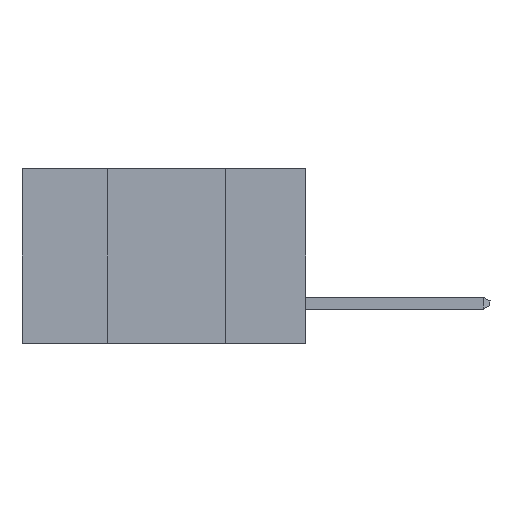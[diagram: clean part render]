
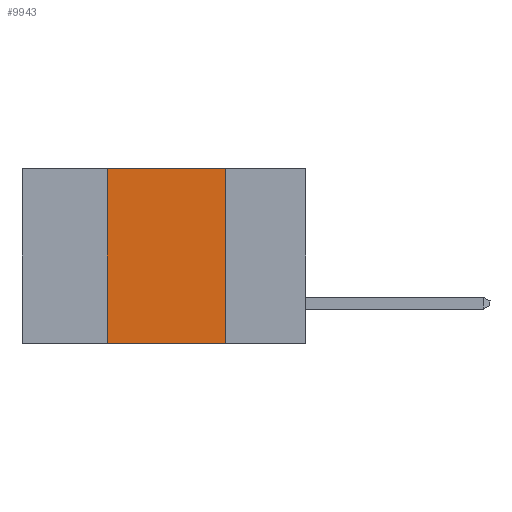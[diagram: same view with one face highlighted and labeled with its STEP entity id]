
A CAD part, left-side view. The second image highlights one B-rep face of the part: STEP entity #9943.
In plain terms, the highlighted planar face has unit normal (-1, 0, 0).
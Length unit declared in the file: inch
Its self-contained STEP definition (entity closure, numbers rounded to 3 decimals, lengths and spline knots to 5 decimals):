
#151 = DIRECTION ( 'NONE',  ( 0., -1., 0. ) ) ;
#464 = EDGE_CURVE ( 'NONE', #7563, #9690, #780, .T. ) ;
#780 = LINE ( 'NONE', #4420, #4636 ) ;
#923 = CARTESIAN_POINT ( 'NONE',  ( 0., 0.17, 0. ) ) ;
#1298 = ORIENTED_EDGE ( 'NONE', *, *, #4960, .F. ) ;
#1433 = EDGE_CURVE ( 'NONE', #7563, #1590, #11849, .T. ) ;
#1549 = CARTESIAN_POINT ( 'NONE',  ( 0., 0.42, -0.37 ) ) ;
#1590 = VERTEX_POINT ( 'NONE', #11187 ) ;
#2091 = AXIS2_PLACEMENT_3D ( 'NONE', #10348, #4934, #11356 ) ;
#2111 = PLANE ( 'NONE',  #2091 ) ;
#2877 = ORIENTED_EDGE ( 'NONE', *, *, #464, .F. ) ;
#3381 = CARTESIAN_POINT ( 'NONE',  ( 0., 0.42, 0. ) ) ;
#3438 = LINE ( 'NONE', #4391, #10645 ) ;
#3635 = VERTEX_POINT ( 'NONE', #923 ) ;
#4286 = VECTOR ( 'NONE', #6633, 39.37008 ) ;
#4391 = CARTESIAN_POINT ( 'NONE',  ( 0., 0.17, -0.37 ) ) ;
#4420 = CARTESIAN_POINT ( 'NONE',  ( 0., 0.42, -0.37 ) ) ;
#4636 = VECTOR ( 'NONE', #9963, 39.37008 ) ;
#4669 = EDGE_CURVE ( 'NONE', #9690, #3635, #11024, .T. ) ;
#4934 = DIRECTION ( 'NONE',  ( 1., 0., 0. ) ) ;
#4960 = EDGE_CURVE ( 'NONE', #3635, #1590, #3438, .T. ) ;
#5655 = ORIENTED_EDGE ( 'NONE', *, *, #1433, .T. ) ;
#6633 = DIRECTION ( 'NONE',  ( 0., -1., 0. ) ) ;
#7159 = DIRECTION ( 'NONE',  ( 0., 0., -1. ) ) ;
#7192 = ORIENTED_EDGE ( 'NONE', *, *, #4669, .F. ) ;
#7563 = VERTEX_POINT ( 'NONE', #1549 ) ;
#7564 = FACE_OUTER_BOUND ( 'NONE', #10898, .T. ) ;
#7581 = CARTESIAN_POINT ( 'NONE',  ( 0., 0.6, 0. ) ) ;
#8067 = VECTOR ( 'NONE', #151, 39.37008 ) ;
#8348 = CARTESIAN_POINT ( 'NONE',  ( 0., 0.6, -0.37 ) ) ;
#9690 = VERTEX_POINT ( 'NONE', #3381 ) ;
#9943 = ADVANCED_FACE ( 'NONE', ( #7564 ), #2111, .F. ) ;
#9963 = DIRECTION ( 'NONE',  ( 0., 0., 1. ) ) ;
#10348 = CARTESIAN_POINT ( 'NONE',  ( 0., 0.6, 0. ) ) ;
#10645 = VECTOR ( 'NONE', #7159, 39.37008 ) ;
#10898 = EDGE_LOOP ( 'NONE', ( #1298, #7192, #2877, #5655 ) ) ;
#11024 = LINE ( 'NONE', #7581, #4286 ) ;
#11187 = CARTESIAN_POINT ( 'NONE',  ( 0., 0.17, -0.37 ) ) ;
#11356 = DIRECTION ( 'NONE',  ( 0., 0., -1. ) ) ;
#11849 = LINE ( 'NONE', #8348, #8067 ) ;
